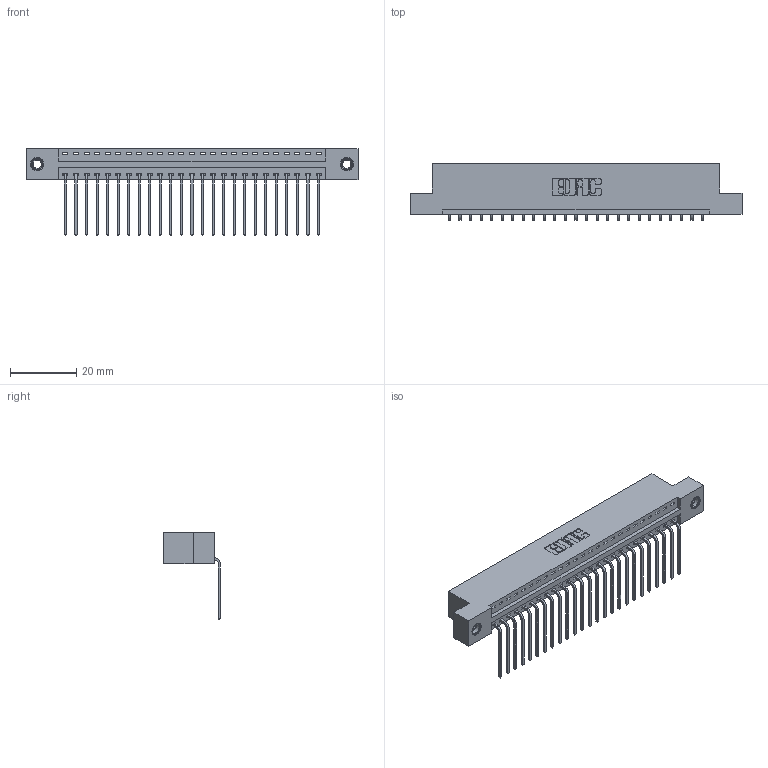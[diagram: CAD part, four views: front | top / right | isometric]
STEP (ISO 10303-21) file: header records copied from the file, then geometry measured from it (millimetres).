
FILE_DESCRIPTION (( 'STEP AP203' ), '1' );
FILE_NAME ('396-025-559-107.STEP', '2019-10-31T21:22:03', ( '' ), ( '' ), 'SwSTEP 2.0', 'SolidWorks 2016', '' );
FILE_SCHEMA (( 'CONFIG_CONTROL_DESIGN' ));
Length unit declared in the file: inch
Products named in the file (4): 396-025-559-107; 346 Part_Flush Mounting Lugs - 0.156 Dia-TI; 345-292-001_558 559 Tail - 1; 345-250-001_345-250-005-103
Assembly tree (28 placements, depth 2):
  396-025-559-107
    346 Part_Flush Mounting Lugs - 0.156 Dia-TI
    345-292-001_558 559 Tail - 1  x25
    345-250-001_345-250-005-103  x2
Bounding box: 99.95 x 17.08 x 26.16 mm (x, y, z)
Volume: 9520 mm3; surface area: 12246.9 mm2
Topology: 28 solids, 28 shells, 1682 faces, 5015 edges, 3302 vertices
Faces by surface type: plane 1158, cylinder 508, cone 12, torus 4
Entity records: 19074 total; most frequent: CARTESIAN_POINT 3258, ORIENTED_EDGE 3210, DIRECTION 2921, EDGE_CURVE 1605, VECTOR 1353, LINE 1353, VERTEX_POINT 1064, AXIS2_PLACEMENT_3D 784
